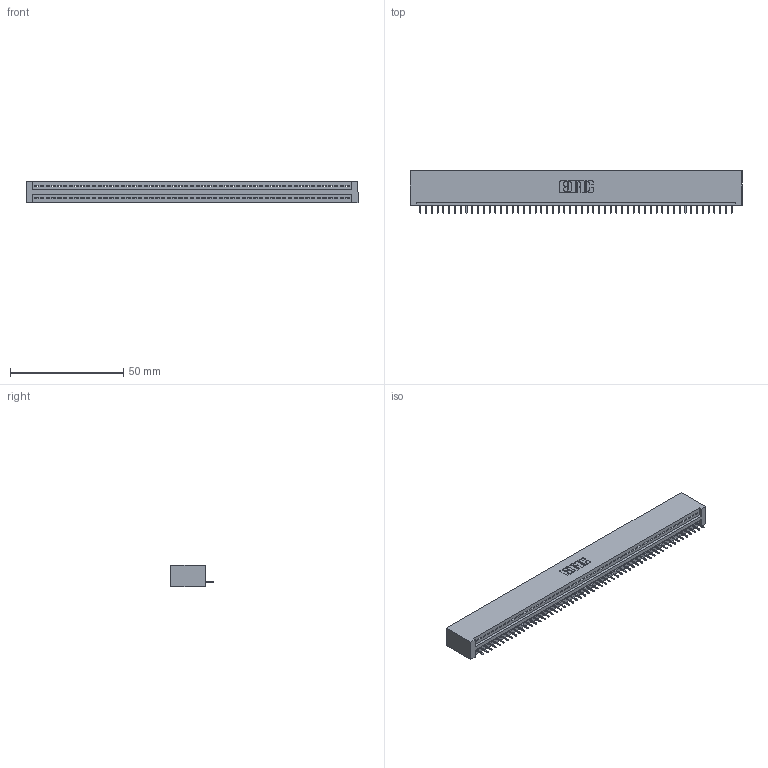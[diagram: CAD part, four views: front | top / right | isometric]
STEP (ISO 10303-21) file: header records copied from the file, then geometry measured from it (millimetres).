
FILE_DESCRIPTION (( 'STEP AP203' ), '1' );
FILE_NAME ('345-055-525-101.STEP', '2020-09-20T17:55:01', ( '' ), ( '' ), 'SwSTEP 2.0', 'SolidWorks 2020', '' );
FILE_SCHEMA (( 'CONFIG_CONTROL_DESIGN' ));
Length unit declared in the file: inch
Products named in the file (3): 345 Part_No Mounting Lugs; 345-292-001_345-293-125; 345-055-525-101
Assembly tree (56 placements, depth 2):
  345-055-525-101
    345 Part_No Mounting Lugs
    345-292-001_345-293-125  x55
Bounding box: 146.3 x 18.72 x 9.4 mm (x, y, z)
Volume: 14362.4 mm3; surface area: 18704.3 mm2
Topology: 56 solids, 56 shells, 3528 faces, 10217 edges, 6590 vertices
Faces by surface type: plane 2606, cylinder 922
Entity records: 39441 total; most frequent: CARTESIAN_POINT 6837, ORIENTED_EDGE 6826, DIRECTION 5947, EDGE_CURVE 3413, LINE 3073, VECTOR 3073, VERTEX_POINT 2270, AXIS2_PLACEMENT_3D 1437
